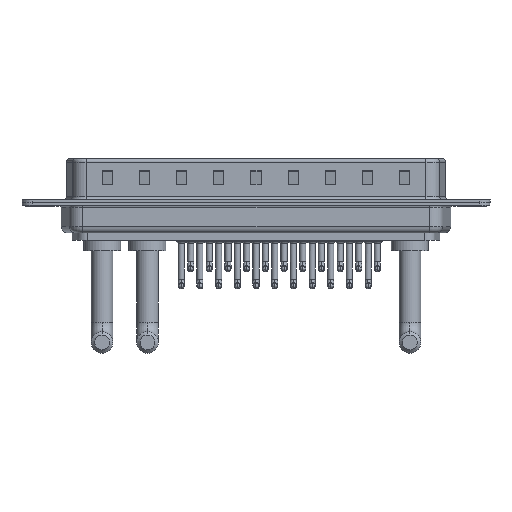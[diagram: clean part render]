
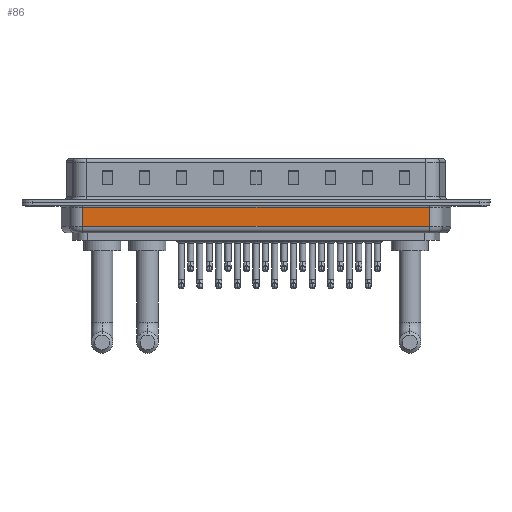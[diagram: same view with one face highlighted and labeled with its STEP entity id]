
A CAD part, front view. The second image highlights one B-rep face of the part: STEP entity #86.
In plain terms, the highlighted planar face has unit normal (0, -1, 0).
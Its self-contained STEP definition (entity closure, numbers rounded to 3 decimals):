
#86 = ADVANCED_FACE ( 'NONE', ( #21628 ), #20259, .F. ) ;
#1279 = ORIENTED_EDGE ( 'NONE', *, *, #18801, .T. ) ;
#1569 = CARTESIAN_POINT ( 'NONE',  ( 6.031, -5.35, -0.65 ) ) ;
#2046 = DIRECTION ( 'NONE',  ( 0., 0., 1. ) ) ;
#2299 = CARTESIAN_POINT ( 'NONE',  ( 6.031, -5.35, -4.5 ) ) ;
#2403 = VERTEX_POINT ( 'NONE', #5802 ) ;
#3223 = VERTEX_POINT ( 'NONE', #9571 ) ;
#5062 = LINE ( 'NONE', #13364, #5383 ) ;
#5383 = VECTOR ( 'NONE', #9266, 1000. ) ;
#5802 = CARTESIAN_POINT ( 'NONE',  ( 57.469, -5.35, -0.65 ) ) ;
#6470 = ORIENTED_EDGE ( 'NONE', *, *, #12360, .T. ) ;
#7765 = DIRECTION ( 'NONE',  ( 0., 1., 0. ) ) ;
#8373 = DIRECTION ( 'NONE',  ( -1., 0., 0. ) ) ;
#9266 = DIRECTION ( 'NONE',  ( 0., 0., 1. ) ) ;
#9571 = CARTESIAN_POINT ( 'NONE',  ( 57.469, -5.35, -3.5 ) ) ;
#10087 = EDGE_CURVE ( 'NONE', #2403, #11643, #10369, .T. ) ;
#10369 = LINE ( 'NONE', #11965, #22900 ) ;
#10967 = DIRECTION ( 'NONE',  ( 1., 0., 0. ) ) ;
#11643 = VERTEX_POINT ( 'NONE', #1569 ) ;
#11963 = LINE ( 'NONE', #14202, #15832 ) ;
#11965 = CARTESIAN_POINT ( 'NONE',  ( 6.031, -5.35, -0.65 ) ) ;
#12050 = VECTOR ( 'NONE', #10967, 1000. ) ;
#12360 = EDGE_CURVE ( 'NONE', #3223, #2403, #5062, .T. ) ;
#12940 = ORIENTED_EDGE ( 'NONE', *, *, #10087, .T. ) ;
#13364 = CARTESIAN_POINT ( 'NONE',  ( 57.469, -5.35, -4.5 ) ) ;
#14202 = CARTESIAN_POINT ( 'NONE',  ( 6.031, -5.35, -4.5 ) ) ;
#15832 = VECTOR ( 'NONE', #2046, 1000. ) ;
#18158 = EDGE_CURVE ( 'NONE', #25692, #11643, #11963, .T. ) ;
#18431 = DIRECTION ( 'NONE',  ( -1., 0., 0. ) ) ;
#18801 = EDGE_CURVE ( 'NONE', #25692, #3223, #24836, .T. ) ;
#18898 = CARTESIAN_POINT ( 'NONE',  ( 6.031, -5.35, -3.5 ) ) ;
#20259 = PLANE ( 'NONE',  #23043 ) ;
#21628 = FACE_OUTER_BOUND ( 'NONE', #25570, .T. ) ;
#22900 = VECTOR ( 'NONE', #18431, 1000. ) ;
#23043 = AXIS2_PLACEMENT_3D ( 'NONE', #2299, #7765, #8373 ) ;
#24836 = LINE ( 'NONE', #18898, #12050 ) ;
#25291 = ORIENTED_EDGE ( 'NONE', *, *, #18158, .F. ) ;
#25570 = EDGE_LOOP ( 'NONE', ( #25291, #1279, #6470, #12940 ) ) ;
#25692 = VERTEX_POINT ( 'NONE', #26008 ) ;
#26008 = CARTESIAN_POINT ( 'NONE',  ( 6.031, -5.35, -3.5 ) ) ;
